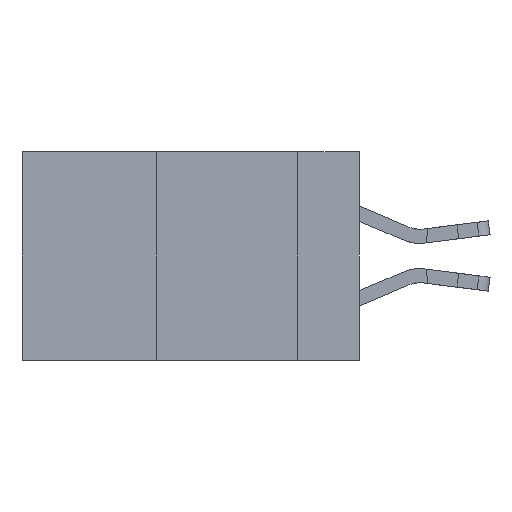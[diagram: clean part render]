
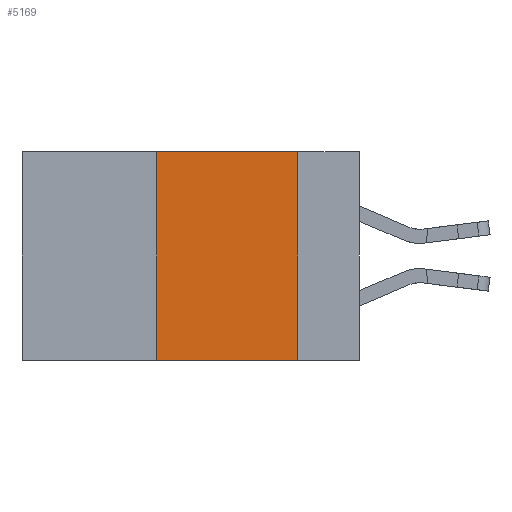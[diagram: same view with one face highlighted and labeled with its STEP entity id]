
A CAD part, left-side view. The second image highlights one B-rep face of the part: STEP entity #5169.
In plain terms, the highlighted planar face has unit normal (-1, 0, 0).
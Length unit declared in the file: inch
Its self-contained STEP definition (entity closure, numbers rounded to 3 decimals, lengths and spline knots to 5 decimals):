
#1474 = LINE ( 'NONE', #2664, #11844 ) ;
#2039 = AXIS2_PLACEMENT_3D ( 'NONE', #25415, #27672, #16586 ) ;
#2664 = CARTESIAN_POINT ( 'NONE',  ( 0., 0.36, 0. ) ) ;
#3330 = EDGE_LOOP ( 'NONE', ( #26275, #10683, #18648, #26937 ) ) ;
#3911 = DIRECTION ( 'NONE',  ( 0., -1., 0. ) ) ;
#4270 = CARTESIAN_POINT ( 'NONE',  ( 0., 0.36, 0. ) ) ;
#4517 = CARTESIAN_POINT ( 'NONE',  ( 0., 0.11, -0.37 ) ) ;
#5131 = CARTESIAN_POINT ( 'NONE',  ( 0., 0.6, 0. ) ) ;
#5169 = ADVANCED_FACE ( 'NONE', ( #18800 ), #16492, .F. ) ;
#5768 = CARTESIAN_POINT ( 'NONE',  ( 0., 0.11, 0. ) ) ;
#6340 = LINE ( 'NONE', #17549, #8397 ) ;
#8397 = VECTOR ( 'NONE', #19839, 39.37008 ) ;
#9340 = VERTEX_POINT ( 'NONE', #16801 ) ;
#10683 = ORIENTED_EDGE ( 'NONE', *, *, #21037, .F. ) ;
#11553 = EDGE_CURVE ( 'NONE', #14330, #20220, #6340, .T. ) ;
#11844 = VECTOR ( 'NONE', #24871, 39.37008 ) ;
#14330 = VERTEX_POINT ( 'NONE', #5768 ) ;
#14426 = VECTOR ( 'NONE', #20253, 39.37008 ) ;
#16492 = PLANE ( 'NONE',  #2039 ) ;
#16586 = DIRECTION ( 'NONE',  ( 0., 0., -1. ) ) ;
#16801 = CARTESIAN_POINT ( 'NONE',  ( 0., 0.36, -0.37 ) ) ;
#17549 = CARTESIAN_POINT ( 'NONE',  ( 0., 0.11, 0. ) ) ;
#18648 = ORIENTED_EDGE ( 'NONE', *, *, #23658, .F. ) ;
#18800 = FACE_OUTER_BOUND ( 'NONE', #3330, .T. ) ;
#18928 = LINE ( 'NONE', #5131, #14426 ) ;
#19839 = DIRECTION ( 'NONE',  ( 0., 0., -1. ) ) ;
#20220 = VERTEX_POINT ( 'NONE', #4517 ) ;
#20253 = DIRECTION ( 'NONE',  ( 0., -1., 0. ) ) ;
#21037 = EDGE_CURVE ( 'NONE', #22260, #14330, #18928, .T. ) ;
#22260 = VERTEX_POINT ( 'NONE', #4270 ) ;
#23426 = CARTESIAN_POINT ( 'NONE',  ( 0., 0.6, -0.37 ) ) ;
#23658 = EDGE_CURVE ( 'NONE', #9340, #22260, #1474, .T. ) ;
#24871 = DIRECTION ( 'NONE',  ( 0., 0., 1. ) ) ;
#25006 = VECTOR ( 'NONE', #3911, 39.37008 ) ;
#25415 = CARTESIAN_POINT ( 'NONE',  ( 0., 0.6, 0. ) ) ;
#26259 = EDGE_CURVE ( 'NONE', #9340, #20220, #27886, .T. ) ;
#26275 = ORIENTED_EDGE ( 'NONE', *, *, #11553, .F. ) ;
#26937 = ORIENTED_EDGE ( 'NONE', *, *, #26259, .T. ) ;
#27672 = DIRECTION ( 'NONE',  ( 1., 0., 0. ) ) ;
#27886 = LINE ( 'NONE', #23426, #25006 ) ;
